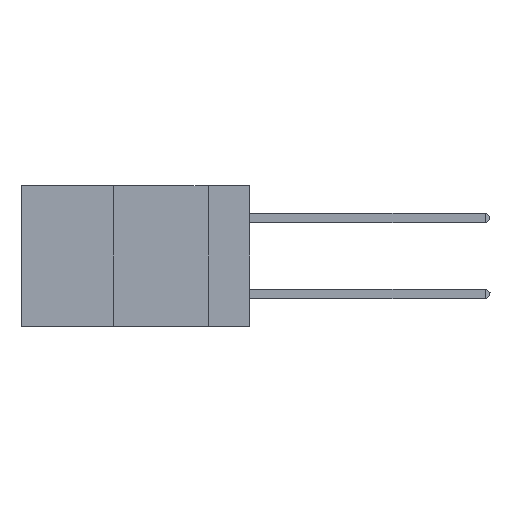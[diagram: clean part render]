
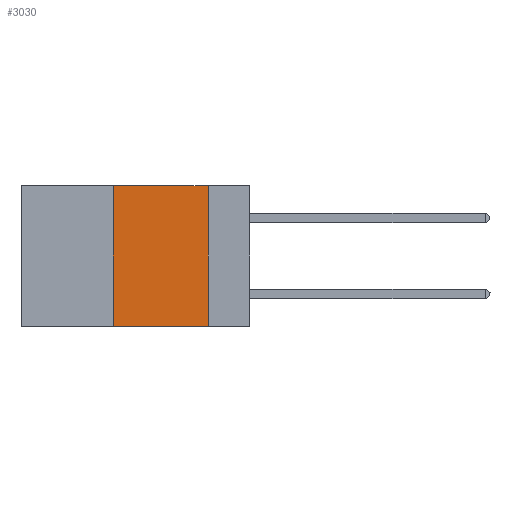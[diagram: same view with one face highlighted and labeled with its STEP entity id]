
A CAD part, left-side view. The second image highlights one B-rep face of the part: STEP entity #3030.
In plain terms, the highlighted planar face has unit normal (-1, 0, 0).
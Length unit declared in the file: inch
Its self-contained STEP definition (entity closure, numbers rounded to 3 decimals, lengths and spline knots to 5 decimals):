
#172 = EDGE_CURVE ( 'NONE', #446, #4242, #14993, .T. ) ;
#446 = VERTEX_POINT ( 'NONE', #14726 ) ;
#702 = CARTESIAN_POINT ( 'NONE',  ( 0., 0.6, 0. ) ) ;
#2321 = ORIENTED_EDGE ( 'NONE', *, *, #16593, .F. ) ;
#2506 = VERTEX_POINT ( 'NONE', #16254 ) ;
#3030 = ADVANCED_FACE ( 'NONE', ( #8791 ), #5154, .F. ) ;
#3457 = DIRECTION ( 'NONE',  ( 1., 0., 0. ) ) ;
#3483 = DIRECTION ( 'NONE',  ( 0., 0., 1. ) ) ;
#3505 = DIRECTION ( 'NONE',  ( 0., 0., -1. ) ) ;
#3891 = EDGE_CURVE ( 'NONE', #19475, #4242, #22082, .T. ) ;
#4046 = CARTESIAN_POINT ( 'NONE',  ( 0., 0.11, 0. ) ) ;
#4113 = DIRECTION ( 'NONE',  ( 0., -1., 0. ) ) ;
#4153 = EDGE_LOOP ( 'NONE', ( #8771, #15673, #2321, #9352 ) ) ;
#4242 = VERTEX_POINT ( 'NONE', #14630 ) ;
#5090 = VECTOR ( 'NONE', #3505, 39.37008 ) ;
#5154 = PLANE ( 'NONE',  #19369 ) ;
#6147 = LINE ( 'NONE', #702, #19160 ) ;
#6694 = CARTESIAN_POINT ( 'NONE',  ( 0., 0.6, -0.37 ) ) ;
#8356 = LINE ( 'NONE', #10078, #17658 ) ;
#8771 = ORIENTED_EDGE ( 'NONE', *, *, #3891, .F. ) ;
#8791 = FACE_OUTER_BOUND ( 'NONE', #4153, .T. ) ;
#9057 = VECTOR ( 'NONE', #22191, 39.37008 ) ;
#9352 = ORIENTED_EDGE ( 'NONE', *, *, #172, .T. ) ;
#10078 = CARTESIAN_POINT ( 'NONE',  ( 0., 0.36, 0. ) ) ;
#14630 = CARTESIAN_POINT ( 'NONE',  ( 0., 0.11, -0.37 ) ) ;
#14726 = CARTESIAN_POINT ( 'NONE',  ( 0., 0.36, -0.37 ) ) ;
#14993 = LINE ( 'NONE', #6694, #9057 ) ;
#15411 = CARTESIAN_POINT ( 'NONE',  ( 0., 0.6, 0. ) ) ;
#15673 = ORIENTED_EDGE ( 'NONE', *, *, #19838, .F. ) ;
#16254 = CARTESIAN_POINT ( 'NONE',  ( 0., 0.36, 0. ) ) ;
#16593 = EDGE_CURVE ( 'NONE', #446, #2506, #8356, .T. ) ;
#17658 = VECTOR ( 'NONE', #3483, 39.37008 ) ;
#19160 = VECTOR ( 'NONE', #4113, 39.37008 ) ;
#19369 = AXIS2_PLACEMENT_3D ( 'NONE', #15411, #3457, #22476 ) ;
#19475 = VERTEX_POINT ( 'NONE', #4046 ) ;
#19838 = EDGE_CURVE ( 'NONE', #2506, #19475, #6147, .T. ) ;
#22082 = LINE ( 'NONE', #22317, #5090 ) ;
#22191 = DIRECTION ( 'NONE',  ( 0., -1., 0. ) ) ;
#22317 = CARTESIAN_POINT ( 'NONE',  ( 0., 0.11, 0. ) ) ;
#22476 = DIRECTION ( 'NONE',  ( 0., 0., -1. ) ) ;
